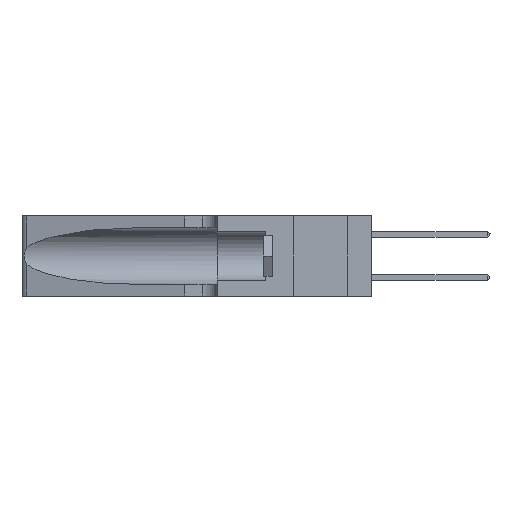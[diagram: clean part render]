
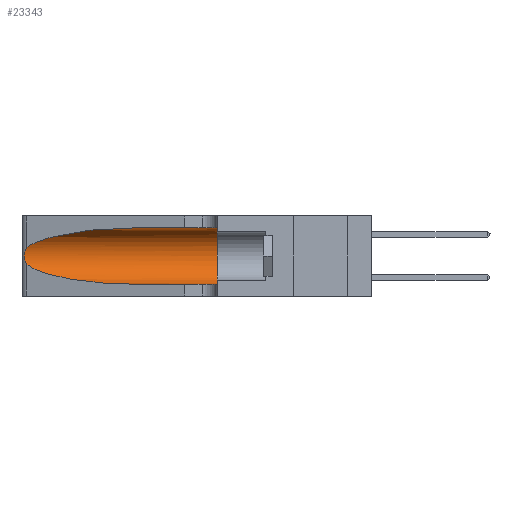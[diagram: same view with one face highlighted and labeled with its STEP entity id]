
A CAD part, left-side view. The second image highlights one B-rep face of the part: STEP entity #23343.
In plain terms, the highlighted cylindrical face has radius 3.308 mm (diameter 6.617 mm), a partial arc.
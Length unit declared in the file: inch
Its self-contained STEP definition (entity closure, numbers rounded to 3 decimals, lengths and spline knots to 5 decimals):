
#89 = CARTESIAN_POINT ( 'NONE',  ( 0.2373, 1.15595, 0.28018 ) ) ;
#146 = CIRCLE ( 'NONE', #21336, 0.13025 ) ;
#669 = LINE ( 'NONE', #7504, #18582 ) ;
#2365 = B_SPLINE_CURVE_WITH_KNOTS ( 'NONE', 3,
 ( #26625, #32024, #15112, #34853, #20825, #3823, #32601, #27984, #30808, #11175, #16835, #19702, #11411, #2730 ),
 .UNSPECIFIED., .F., .F.,
 ( 4, 2, 2, 2, 2, 2, 4 ),
 ( 0., 0.00027, 0.00053, 0.00107, 0.0016, 0.00187, 0.00214 ),
 .UNSPECIFIED. ) ;
#2730 = CARTESIAN_POINT ( 'NONE',  ( 0.25487, 1.22718, 0.14631 ) ) ;
#3823 = CARTESIAN_POINT ( 'NONE',  ( 0.26018, 1.23835, 0.19895 ) ) ;
#4008 = EDGE_CURVE ( 'NONE', #36039, #27473, #10773, .T. ) ;
#4091 = CARTESIAN_POINT ( 'NONE',  ( 0.1305, 0.35, 0.185 ) ) ;
#4493 = EDGE_CURVE ( 'NONE', #15871, #36039, #2365, .T. ) ;
#4914 = CARTESIAN_POINT ( 'NONE',  ( 0.18966, 0.96281, 0.05475 ) ) ;
#5387 = CARTESIAN_POINT ( 'NONE',  ( 0.25487, 1.22718, 0.22369 ) ) ;
#5500 = CARTESIAN_POINT ( 'NONE',  ( 0.18966, 0.96281, 0.31525 ) ) ;
#6836 = DIRECTION ( 'NONE',  ( 0., 0., 1. ) ) ;
#6877 = ORIENTED_EDGE ( 'NONE', *, *, #30650, .F. ) ;
#7453 = CARTESIAN_POINT ( 'NONE',  ( 0.1305, 0.72297, 0.31525 ) ) ;
#7504 = CARTESIAN_POINT ( 'NONE',  ( 0.1305, 1.61858, 0.05475 ) ) ;
#10773 =( BOUNDED_CURVE ( )  B_SPLINE_CURVE ( 3, ( #13241, #21901, #4914, #22369 ),
 .UNSPECIFIED., .F., .F. ) 
 B_SPLINE_CURVE_WITH_KNOTS ( ( 4, 4 ),
 ( 3.44316, 4.71239 ),
 .UNSPECIFIED. ) 
 CURVE ( )  GEOMETRIC_REPRESENTATION_ITEM ( )  RATIONAL_B_SPLINE_CURVE ( ( 1., 0.87, 0.87, 1. ) ) 
 REPRESENTATION_ITEM ( '' )  );
#11175 = CARTESIAN_POINT ( 'NONE',  ( 0.25856, 1.23593, 0.16098 ) ) ;
#11411 = CARTESIAN_POINT ( 'NONE',  ( 0.25555, 1.22993, 0.14849 ) ) ;
#11967 = AXIS2_PLACEMENT_3D ( 'NONE', #32226, #34814, #12134 ) ;
#12134 = DIRECTION ( 'NONE',  ( 0., 0., -1. ) ) ;
#12813 = ORIENTED_EDGE ( 'NONE', *, *, #30645, .F. ) ;
#13241 = CARTESIAN_POINT ( 'NONE',  ( 0.25487, 1.22718, 0.14631 ) ) ;
#14161 = CARTESIAN_POINT ( 'NONE',  ( 0.1305, 0.35, 0.31525 ) ) ;
#15112 = CARTESIAN_POINT ( 'NONE',  ( 0.25639, 1.23184, 0.21858 ) ) ;
#15279 = EDGE_CURVE ( 'NONE', #34645, #15871, #29812, .T. ) ;
#15871 = VERTEX_POINT ( 'NONE', #24782 ) ;
#16835 = CARTESIAN_POINT ( 'NONE',  ( 0.25789, 1.23486, 0.15765 ) ) ;
#17010 = CARTESIAN_POINT ( 'NONE',  ( 0.1305, 0.72297, 0.31525 ) ) ;
#18582 = VECTOR ( 'NONE', #20632, 39.37008 ) ;
#19412 = VERTEX_POINT ( 'NONE', #14161 ) ;
#19702 = CARTESIAN_POINT ( 'NONE',  ( 0.25639, 1.23186, 0.15144 ) ) ;
#20632 = DIRECTION ( 'NONE',  ( 0., -1., 0. ) ) ;
#20825 = CARTESIAN_POINT ( 'NONE',  ( 0.25854, 1.2359, 0.20912 ) ) ;
#21336 = AXIS2_PLACEMENT_3D ( 'NONE', #4091, #34739, #6836 ) ;
#21591 = FACE_OUTER_BOUND ( 'NONE', #36364, .T. ) ;
#21844 = VECTOR ( 'NONE', #23665, 39.37008 ) ;
#21901 = CARTESIAN_POINT ( 'NONE',  ( 0.2373, 1.15595, 0.08982 ) ) ;
#22369 = CARTESIAN_POINT ( 'NONE',  ( 0.1305, 0.72297, 0.05475 ) ) ;
#22622 = ORIENTED_EDGE ( 'NONE', *, *, #27120, .T. ) ;
#23343 = ADVANCED_FACE ( 'NONE', ( #21591 ), #34781, .F. ) ;
#23665 = DIRECTION ( 'NONE',  ( 0., -1., 0. ) ) ;
#24079 = ORIENTED_EDGE ( 'NONE', *, *, #4493, .T. ) ;
#24782 = CARTESIAN_POINT ( 'NONE',  ( 0.25487, 1.22718, 0.22369 ) ) ;
#26625 = CARTESIAN_POINT ( 'NONE',  ( 0.25487, 1.22718, 0.22369 ) ) ;
#27114 = ORIENTED_EDGE ( 'NONE', *, *, #15279, .T. ) ;
#27120 = EDGE_CURVE ( 'NONE', #27473, #32563, #669, .T. ) ;
#27473 = VERTEX_POINT ( 'NONE', #31323 ) ;
#27984 = CARTESIAN_POINT ( 'NONE',  ( 0.26075, 1.23896, 0.178 ) ) ;
#28037 = LINE ( 'NONE', #32037, #21844 ) ;
#29812 =( BOUNDED_CURVE ( )  B_SPLINE_CURVE ( 3, ( #17010, #5500, #89, #5387 ),
 .UNSPECIFIED., .F., .T. ) 
 B_SPLINE_CURVE_WITH_KNOTS ( ( 4, 4 ),
 ( 1.5708, 2.84003 ),
 .UNSPECIFIED. ) 
 CURVE ( )  GEOMETRIC_REPRESENTATION_ITEM ( )  RATIONAL_B_SPLINE_CURVE ( ( 1., 0.87, 0.87, 1. ) ) 
 REPRESENTATION_ITEM ( '' )  );
#30645 = EDGE_CURVE ( 'NONE', #34645, #19412, #28037, .T. ) ;
#30650 = EDGE_CURVE ( 'NONE', #19412, #32563, #146, .T. ) ;
#30808 = CARTESIAN_POINT ( 'NONE',  ( 0.26017, 1.23833, 0.17102 ) ) ;
#31323 = CARTESIAN_POINT ( 'NONE',  ( 0.1305, 0.72297, 0.05475 ) ) ;
#31863 = ORIENTED_EDGE ( 'NONE', *, *, #4008, .T. ) ;
#32024 = CARTESIAN_POINT ( 'NONE',  ( 0.25555, 1.22994, 0.2215 ) ) ;
#32037 = CARTESIAN_POINT ( 'NONE',  ( 0.1305, 1.61858, 0.31525 ) ) ;
#32226 = CARTESIAN_POINT ( 'NONE',  ( 0.1305, 1.61858, 0.185 ) ) ;
#32563 = VERTEX_POINT ( 'NONE', #34636 ) ;
#32601 = CARTESIAN_POINT ( 'NONE',  ( 0.26075, 1.23896, 0.19203 ) ) ;
#34636 = CARTESIAN_POINT ( 'NONE',  ( 0.1305, 0.35, 0.05475 ) ) ;
#34645 = VERTEX_POINT ( 'NONE', #7453 ) ;
#34739 = DIRECTION ( 'NONE',  ( 0., 1., 0. ) ) ;
#34781 = CYLINDRICAL_SURFACE ( 'NONE', #11967, 0.13025 ) ;
#34814 = DIRECTION ( 'NONE',  ( 0., -1., 0. ) ) ;
#34853 = CARTESIAN_POINT ( 'NONE',  ( 0.25787, 1.23484, 0.2124 ) ) ;
#35165 = CARTESIAN_POINT ( 'NONE',  ( 0.25487, 1.22718, 0.14631 ) ) ;
#36039 = VERTEX_POINT ( 'NONE', #35165 ) ;
#36364 = EDGE_LOOP ( 'NONE', ( #27114, #24079, #31863, #22622, #6877, #12813 ) ) ;
